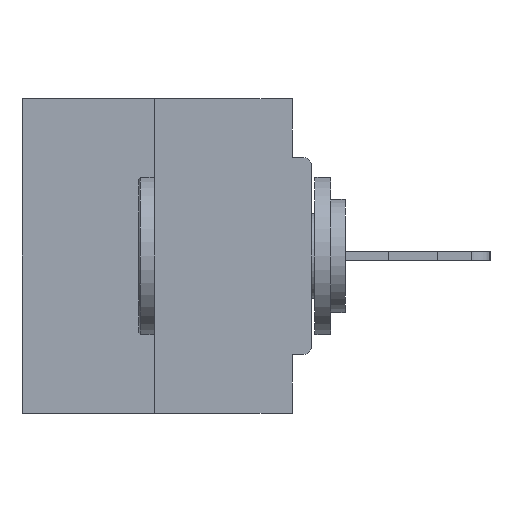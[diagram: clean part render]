
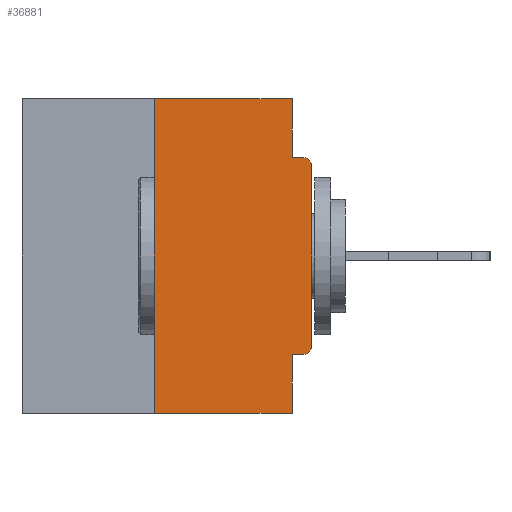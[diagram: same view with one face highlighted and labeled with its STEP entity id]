
A CAD part, left-side view. The second image highlights one B-rep face of the part: STEP entity #36881.
In plain terms, the highlighted planar face has unit normal (-1, 0, 0).
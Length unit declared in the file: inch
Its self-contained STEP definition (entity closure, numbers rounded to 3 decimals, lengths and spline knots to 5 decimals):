
#307 = LINE ( 'NONE', #29805, #37702 ) ;
#1040 = CARTESIAN_POINT ( 'NONE',  ( 0., 0.031, -0.5 ) ) ;
#2364 = DIRECTION ( 'NONE',  ( 0., 0., -1. ) ) ;
#2617 = LINE ( 'NONE', #3017, #23305 ) ;
#2848 = CARTESIAN_POINT ( 'NONE',  ( 0., 0.031, -0.0935 ) ) ;
#2877 = VERTEX_POINT ( 'NONE', #20691 ) ;
#3017 = CARTESIAN_POINT ( 'NONE',  ( 0., 0.46, -0.5 ) ) ;
#3359 = VERTEX_POINT ( 'NONE', #15803 ) ;
#3604 = DIRECTION ( 'NONE',  ( 0., 0., -1. ) ) ;
#5396 = VERTEX_POINT ( 'NONE', #2848 ) ;
#6008 = EDGE_CURVE ( 'NONE', #17339, #12228, #35927, .T. ) ;
#6048 = VECTOR ( 'NONE', #28472, 39.37008 ) ;
#6394 = FACE_OUTER_BOUND ( 'NONE', #30422, .T. ) ;
#8535 = AXIS2_PLACEMENT_3D ( 'NONE', #24142, #15732, #36754 ) ;
#9306 = VECTOR ( 'NONE', #11503, 39.37008 ) ;
#9366 = VERTEX_POINT ( 'NONE', #18656 ) ;
#9906 = LINE ( 'NONE', #19107, #24346 ) ;
#10028 = DIRECTION ( 'NONE',  ( 0., 0., -1. ) ) ;
#10366 = CARTESIAN_POINT ( 'NONE',  ( 0., 0., -0.4065 ) ) ;
#11503 = DIRECTION ( 'NONE',  ( 0., 0., -1. ) ) ;
#11720 = VERTEX_POINT ( 'NONE', #21381 ) ;
#11837 = CARTESIAN_POINT ( 'NONE',  ( 0., 0.015, -0.4065 ) ) ;
#12142 = AXIS2_PLACEMENT_3D ( 'NONE', #31035, #12811, #3604 ) ;
#12181 = CARTESIAN_POINT ( 'NONE',  ( 0., 0.031, 0. ) ) ;
#12228 = VERTEX_POINT ( 'NONE', #1040 ) ;
#12584 = ORIENTED_EDGE ( 'NONE', *, *, #21444, .T. ) ;
#12811 = DIRECTION ( 'NONE',  ( 1., 0., 0. ) ) ;
#15732 = DIRECTION ( 'NONE',  ( -1., 0., 0. ) ) ;
#15803 = CARTESIAN_POINT ( 'NONE',  ( 0., 0.25, -0.5 ) ) ;
#16258 = CARTESIAN_POINT ( 'NONE',  ( 0., 0., -0.0935 ) ) ;
#17339 = VERTEX_POINT ( 'NONE', #21782 ) ;
#18656 = CARTESIAN_POINT ( 'NONE',  ( 0., 0., -0.1085 ) ) ;
#18838 = PLANE ( 'NONE',  #12142 ) ;
#18923 = DIRECTION ( 'NONE',  ( 0., 0., 1. ) ) ;
#19107 = CARTESIAN_POINT ( 'NONE',  ( 0., 0., 0. ) ) ;
#19443 = DIRECTION ( 'NONE',  ( -1., 0., 0. ) ) ;
#19648 = LINE ( 'NONE', #16258, #6048 ) ;
#20270 = ORIENTED_EDGE ( 'NONE', *, *, #20301, .T. ) ;
#20301 = EDGE_CURVE ( 'NONE', #29995, #11720, #23272, .T. ) ;
#20583 = CARTESIAN_POINT ( 'NONE',  ( 0., 0.25, 0. ) ) ;
#20691 = CARTESIAN_POINT ( 'NONE',  ( 0., 0.015, -0.0935 ) ) ;
#21003 = EDGE_CURVE ( 'NONE', #3359, #34000, #22873, .T. ) ;
#21163 = ORIENTED_EDGE ( 'NONE', *, *, #21003, .F. ) ;
#21190 = EDGE_CURVE ( 'NONE', #3359, #12228, #2617, .T. ) ;
#21255 = DIRECTION ( 'NONE',  ( 0., -1., 0. ) ) ;
#21381 = CARTESIAN_POINT ( 'NONE',  ( 0., 0., -0.3915 ) ) ;
#21444 = EDGE_CURVE ( 'NONE', #9366, #2877, #27794, .T. ) ;
#21748 = VERTEX_POINT ( 'NONE', #12181 ) ;
#21782 = CARTESIAN_POINT ( 'NONE',  ( 0., 0.031, -0.4065 ) ) ;
#22381 = DIRECTION ( 'NONE',  ( 0., 1., 0. ) ) ;
#22610 = CARTESIAN_POINT ( 'NONE',  ( 0., 0.031, -0.5 ) ) ;
#22780 = ORIENTED_EDGE ( 'NONE', *, *, #6008, .F. ) ;
#22873 = LINE ( 'NONE', #32273, #30946 ) ;
#23272 = CIRCLE ( 'NONE', #8535, 0.015 ) ;
#23305 = VECTOR ( 'NONE', #21255, 39.37008 ) ;
#23914 = EDGE_CURVE ( 'NONE', #11720, #9366, #9906, .T. ) ;
#24142 = CARTESIAN_POINT ( 'NONE',  ( 0., 0.015, -0.3915 ) ) ;
#24346 = VECTOR ( 'NONE', #18923, 39.37008 ) ;
#25125 = ORIENTED_EDGE ( 'NONE', *, *, #34025, .F. ) ;
#25910 = VECTOR ( 'NONE', #31985, 39.37008 ) ;
#26010 = EDGE_CURVE ( 'NONE', #29995, #17339, #34969, .T. ) ;
#26077 = DIRECTION ( 'NONE',  ( 0., 0., 1. ) ) ;
#26514 = AXIS2_PLACEMENT_3D ( 'NONE', #34640, #19443, #10028 ) ;
#27794 = CIRCLE ( 'NONE', #26514, 0.015 ) ;
#28472 = DIRECTION ( 'NONE',  ( 0., -1., 0. ) ) ;
#28995 = ORIENTED_EDGE ( 'NONE', *, *, #23914, .T. ) ;
#29400 = VECTOR ( 'NONE', #22381, 39.37008 ) ;
#29805 = CARTESIAN_POINT ( 'NONE',  ( 0., 0.031, 0. ) ) ;
#29995 = VERTEX_POINT ( 'NONE', #11837 ) ;
#30333 = ORIENTED_EDGE ( 'NONE', *, *, #21190, .T. ) ;
#30422 = EDGE_LOOP ( 'NONE', ( #25125, #21163, #30333, #22780, #37411, #20270, #28995, #12584, #37184, #32396 ) ) ;
#30946 = VECTOR ( 'NONE', #26077, 39.37008 ) ;
#31035 = CARTESIAN_POINT ( 'NONE',  ( 0., 0.46, 0. ) ) ;
#31985 = DIRECTION ( 'NONE',  ( 0., -1., 0. ) ) ;
#32273 = CARTESIAN_POINT ( 'NONE',  ( 0., 0.25, 0. ) ) ;
#32396 = ORIENTED_EDGE ( 'NONE', *, *, #37092, .F. ) ;
#32776 = CARTESIAN_POINT ( 'NONE',  ( 0., 0.46, 0. ) ) ;
#33580 = EDGE_CURVE ( 'NONE', #5396, #2877, #19648, .T. ) ;
#34000 = VERTEX_POINT ( 'NONE', #20583 ) ;
#34025 = EDGE_CURVE ( 'NONE', #34000, #21748, #34987, .T. ) ;
#34640 = CARTESIAN_POINT ( 'NONE',  ( 0., 0.015, -0.1085 ) ) ;
#34969 = LINE ( 'NONE', #10366, #29400 ) ;
#34987 = LINE ( 'NONE', #32776, #25910 ) ;
#35927 = LINE ( 'NONE', #22610, #9306 ) ;
#36754 = DIRECTION ( 'NONE',  ( 0., 0., -1. ) ) ;
#36881 = ADVANCED_FACE ( 'NONE', ( #6394 ), #18838, .F. ) ;
#37092 = EDGE_CURVE ( 'NONE', #21748, #5396, #307, .T. ) ;
#37184 = ORIENTED_EDGE ( 'NONE', *, *, #33580, .F. ) ;
#37411 = ORIENTED_EDGE ( 'NONE', *, *, #26010, .F. ) ;
#37702 = VECTOR ( 'NONE', #2364, 39.37008 ) ;
